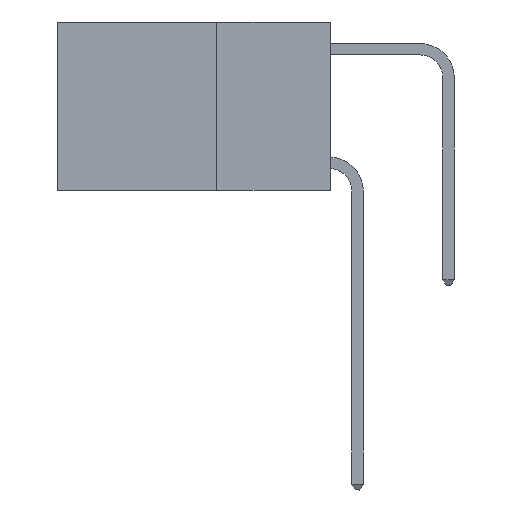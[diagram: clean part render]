
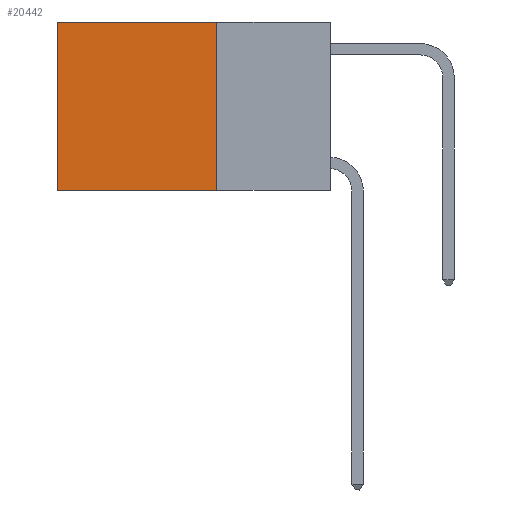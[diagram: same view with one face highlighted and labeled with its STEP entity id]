
A CAD part, left-side view. The second image highlights one B-rep face of the part: STEP entity #20442.
In plain terms, the highlighted planar face has unit normal (-1, 0, 0).
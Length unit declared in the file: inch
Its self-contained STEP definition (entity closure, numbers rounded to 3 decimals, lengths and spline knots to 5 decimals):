
#494 = VERTEX_POINT ( 'NONE', #18719 ) ;
#559 = LINE ( 'NONE', #4978, #17076 ) ;
#3723 = CARTESIAN_POINT ( 'NONE',  ( 0.2625, 0.25, 0. ) ) ;
#3757 = EDGE_CURVE ( 'NONE', #8395, #18138, #8959, .T. ) ;
#4978 = CARTESIAN_POINT ( 'NONE',  ( 0.2625, 0.25, 0. ) ) ;
#5590 = ORIENTED_EDGE ( 'NONE', *, *, #3757, .T. ) ;
#5901 = EDGE_LOOP ( 'NONE', ( #5590, #18045, #11384, #9815 ) ) ;
#5934 = EDGE_CURVE ( 'NONE', #12350, #494, #28040, .T. ) ;
#6216 = CARTESIAN_POINT ( 'NONE',  ( 0.2625, 0.6, 0. ) ) ;
#7107 = DIRECTION ( 'NONE',  ( 0., 1., 0. ) ) ;
#8395 = VERTEX_POINT ( 'NONE', #25054 ) ;
#8567 = PLANE ( 'NONE',  #29308 ) ;
#8959 = LINE ( 'NONE', #6216, #29216 ) ;
#9815 = ORIENTED_EDGE ( 'NONE', *, *, #28090, .T. ) ;
#10722 = FACE_OUTER_BOUND ( 'NONE', #5901, .T. ) ;
#11384 = ORIENTED_EDGE ( 'NONE', *, *, #5934, .F. ) ;
#12292 = CARTESIAN_POINT ( 'NONE',  ( 0.2625, 0.6, -0.37 ) ) ;
#12350 = VERTEX_POINT ( 'NONE', #3723 ) ;
#13020 = DIRECTION ( 'NONE',  ( 1., 0., 0. ) ) ;
#15701 = DIRECTION ( 'NONE',  ( 0., 0., -1. ) ) ;
#16569 = CARTESIAN_POINT ( 'NONE',  ( 0.2625, 0.25, 0. ) ) ;
#17076 = VECTOR ( 'NONE', #7107, 39.37008 ) ;
#17903 = CARTESIAN_POINT ( 'NONE',  ( 0.2625, 0.25, 0. ) ) ;
#18045 = ORIENTED_EDGE ( 'NONE', *, *, #20969, .F. ) ;
#18138 = VERTEX_POINT ( 'NONE', #12292 ) ;
#18577 = VECTOR ( 'NONE', #25062, 39.37008 ) ;
#18719 = CARTESIAN_POINT ( 'NONE',  ( 0.2625, 0.25, -0.37 ) ) ;
#20442 = ADVANCED_FACE ( 'NONE', ( #10722 ), #8567, .F. ) ;
#20969 = EDGE_CURVE ( 'NONE', #494, #18138, #24457, .T. ) ;
#21172 = VECTOR ( 'NONE', #24724, 39.37008 ) ;
#22584 = CARTESIAN_POINT ( 'NONE',  ( 0.2625, 0.25, -0.37 ) ) ;
#24457 = LINE ( 'NONE', #22584, #18577 ) ;
#24724 = DIRECTION ( 'NONE',  ( 0., 0., -1. ) ) ;
#25054 = CARTESIAN_POINT ( 'NONE',  ( 0.2625, 0.6, 0. ) ) ;
#25062 = DIRECTION ( 'NONE',  ( 0., 1., 0. ) ) ;
#27535 = DIRECTION ( 'NONE',  ( 0., 0., -1. ) ) ;
#28040 = LINE ( 'NONE', #16569, #21172 ) ;
#28090 = EDGE_CURVE ( 'NONE', #12350, #8395, #559, .T. ) ;
#29216 = VECTOR ( 'NONE', #15701, 39.37008 ) ;
#29308 = AXIS2_PLACEMENT_3D ( 'NONE', #17903, #13020, #27535 ) ;
